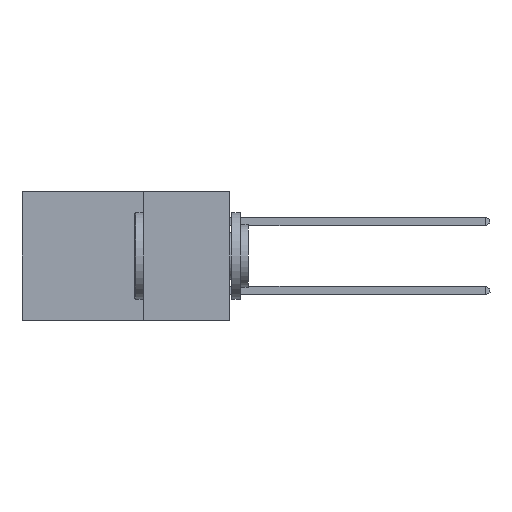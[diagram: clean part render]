
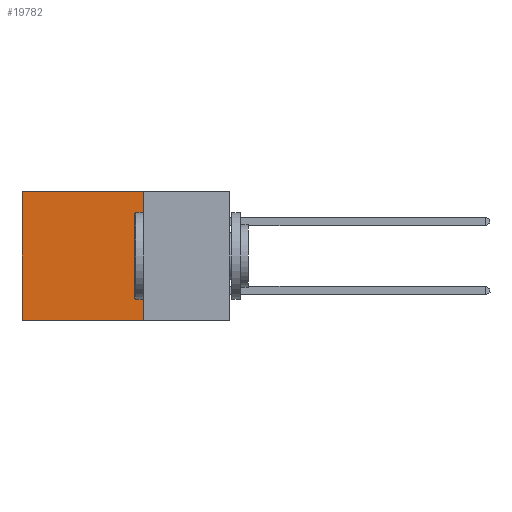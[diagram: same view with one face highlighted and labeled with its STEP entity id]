
A CAD part, left-side view. The second image highlights one B-rep face of the part: STEP entity #19782.
In plain terms, the highlighted planar face has unit normal (-1, 0, 0).
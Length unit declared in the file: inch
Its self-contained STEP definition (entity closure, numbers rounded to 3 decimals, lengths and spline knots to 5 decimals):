
#77 = CARTESIAN_POINT ( 'NONE',  ( 0.298, 0.6, 0. ) ) ;
#336 = VERTEX_POINT ( 'NONE', #77 ) ;
#359 = DIRECTION ( 'NONE',  ( 0., 1., 0. ) ) ;
#1415 = VECTOR ( 'NONE', #11570, 39.37008 ) ;
#2698 = VERTEX_POINT ( 'NONE', #4407 ) ;
#3475 = FACE_OUTER_BOUND ( 'NONE', #9853, .T. ) ;
#4407 = CARTESIAN_POINT ( 'NONE',  ( 0.298, 0.25, -0.37 ) ) ;
#4666 = AXIS2_PLACEMENT_3D ( 'NONE', #17223, #5259, #7157 ) ;
#5259 = DIRECTION ( 'NONE',  ( 1., 0., 0. ) ) ;
#6251 = LINE ( 'NONE', #25037, #19738 ) ;
#7065 = PLANE ( 'NONE',  #4666 ) ;
#7157 = DIRECTION ( 'NONE',  ( 0., 0., -1. ) ) ;
#8742 = EDGE_CURVE ( 'NONE', #336, #9912, #23149, .T. ) ;
#9074 = CARTESIAN_POINT ( 'NONE',  ( 0.298, 0.25, -0.37 ) ) ;
#9853 = EDGE_LOOP ( 'NONE', ( #22954, #20108, #20699, #25377 ) ) ;
#9912 = VERTEX_POINT ( 'NONE', #21433 ) ;
#10359 = VECTOR ( 'NONE', #13203, 39.37008 ) ;
#11570 = DIRECTION ( 'NONE',  ( 0., 0., -1. ) ) ;
#13156 = EDGE_CURVE ( 'NONE', #2698, #9912, #18407, .T. ) ;
#13203 = DIRECTION ( 'NONE',  ( 0., 1., 0. ) ) ;
#13415 = DIRECTION ( 'NONE',  ( 0., 0., -1. ) ) ;
#13446 = CARTESIAN_POINT ( 'NONE',  ( 0.298, 0.25, 0. ) ) ;
#16097 = VECTOR ( 'NONE', #13415, 39.37008 ) ;
#16538 = LINE ( 'NONE', #13446, #1415 ) ;
#17223 = CARTESIAN_POINT ( 'NONE',  ( 0.298, 0.25, 0. ) ) ;
#17935 = CARTESIAN_POINT ( 'NONE',  ( 0.298, 0.25, 0. ) ) ;
#18407 = LINE ( 'NONE', #9074, #10359 ) ;
#19738 = VECTOR ( 'NONE', #359, 39.37008 ) ;
#19782 = ADVANCED_FACE ( 'NONE', ( #3475 ), #7065, .F. ) ;
#20108 = ORIENTED_EDGE ( 'NONE', *, *, #13156, .F. ) ;
#20699 = ORIENTED_EDGE ( 'NONE', *, *, #26307, .F. ) ;
#20797 = VERTEX_POINT ( 'NONE', #17935 ) ;
#21433 = CARTESIAN_POINT ( 'NONE',  ( 0.298, 0.6, -0.37 ) ) ;
#21593 = EDGE_CURVE ( 'NONE', #20797, #336, #6251, .T. ) ;
#22954 = ORIENTED_EDGE ( 'NONE', *, *, #8742, .T. ) ;
#23149 = LINE ( 'NONE', #23733, #16097 ) ;
#23733 = CARTESIAN_POINT ( 'NONE',  ( 0.298, 0.6, 0. ) ) ;
#25037 = CARTESIAN_POINT ( 'NONE',  ( 0.298, 0.25, 0. ) ) ;
#25377 = ORIENTED_EDGE ( 'NONE', *, *, #21593, .T. ) ;
#26307 = EDGE_CURVE ( 'NONE', #20797, #2698, #16538, .T. ) ;
